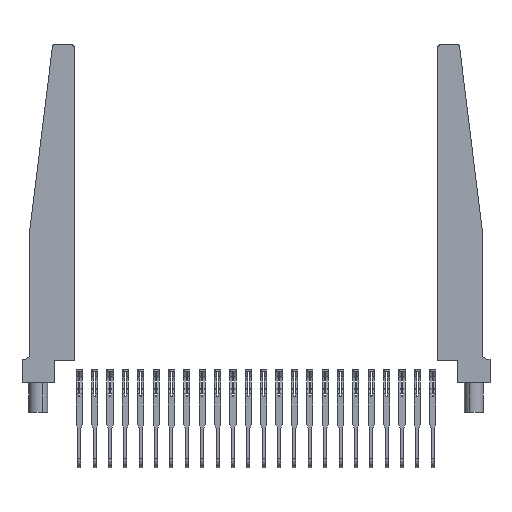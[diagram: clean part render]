
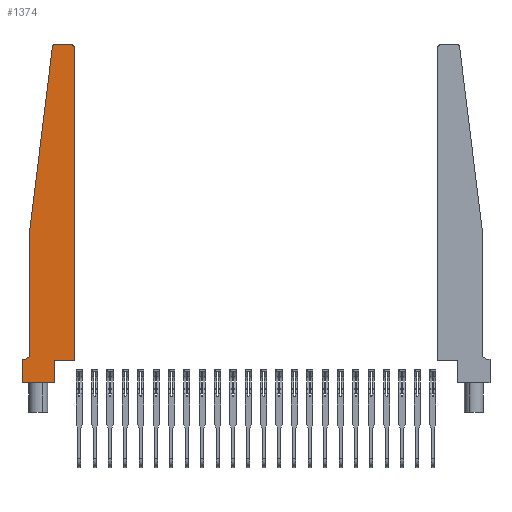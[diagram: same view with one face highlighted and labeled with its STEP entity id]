
A CAD part, top view. The second image highlights one B-rep face of the part: STEP entity #1374.
In plain terms, the highlighted planar face has unit normal (0, 0, 1).
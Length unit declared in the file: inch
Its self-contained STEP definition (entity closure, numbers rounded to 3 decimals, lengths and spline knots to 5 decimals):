
#217 = ORIENTED_EDGE ( 'NONE', *, *, #5809, .T. ) ;
#319 = LINE ( 'NONE', #12160, #12719 ) ;
#435 = CIRCLE ( 'NONE', #21368, 0.03 ) ;
#450 = EDGE_CURVE ( 'NONE', #17572, #12977, #7621, .T. ) ;
#714 = DIRECTION ( 'NONE',  ( -1., 0., 0. ) ) ;
#967 = VERTEX_POINT ( 'NONE', #6766 ) ;
#1080 = DIRECTION ( 'NONE',  ( 1., 0., 0. ) ) ;
#1260 = DIRECTION ( 'NONE',  ( 0., -1., 0. ) ) ;
#1374 = ADVANCED_FACE ( 'NONE', ( #8361 ), #20442, .T. ) ;
#1452 = DIRECTION ( 'NONE',  ( 1., 0., 0. ) ) ;
#1830 = CARTESIAN_POINT ( 'NONE',  ( 0.015, 0.2375, 0.37 ) ) ;
#2026 = ORIENTED_EDGE ( 'NONE', *, *, #15828, .T. ) ;
#2088 = DIRECTION ( 'NONE',  ( -1., 0., 0. ) ) ;
#2246 = CARTESIAN_POINT ( 'NONE',  ( 0.065, 1.25, 0.37 ) ) ;
#2315 = CARTESIAN_POINT ( 'NONE',  ( 0.065, 0.1875, 0.37 ) ) ;
#2542 = VECTOR ( 'NONE', #1260, 39.37008 ) ;
#2791 = LINE ( 'NONE', #9818, #12772 ) ;
#2823 = LINE ( 'NONE', #18687, #9390 ) ;
#3141 = EDGE_CURVE ( 'NONE', #12977, #4894, #17207, .T. ) ;
#3918 = VERTEX_POINT ( 'NONE', #22026 ) ;
#4113 = EDGE_CURVE ( 'NONE', #21723, #4563, #15552, .T. ) ;
#4232 = AXIS2_PLACEMENT_3D ( 'NONE', #1830, #17816, #5049 ) ;
#4384 = ORIENTED_EDGE ( 'NONE', *, *, #6050, .T. ) ;
#4492 = DIRECTION ( 'NONE',  ( 0., 0., 1. ) ) ;
#4563 = VERTEX_POINT ( 'NONE', #21632 ) ;
#4652 = ORIENTED_EDGE ( 'NONE', *, *, #8075, .T. ) ;
#4852 = AXIS2_PLACEMENT_3D ( 'NONE', #13099, #16649, #6331 ) ;
#4894 = VERTEX_POINT ( 'NONE', #12355 ) ;
#5049 = DIRECTION ( 'NONE',  ( -1., 0., 0. ) ) ;
#5094 = DIRECTION ( 'NONE',  ( 1., 0., 0. ) ) ;
#5099 = EDGE_CURVE ( 'NONE', #4563, #3918, #10630, .T. ) ;
#5234 = DIRECTION ( 'NONE',  ( -0.122, -0.992, 0. ) ) ;
#5555 = LINE ( 'NONE', #17849, #11280 ) ;
#5809 = EDGE_CURVE ( 'NONE', #21485, #18608, #18419, .T. ) ;
#6050 = EDGE_CURVE ( 'NONE', #19010, #16733, #435, .T. ) ;
#6229 = ORIENTED_EDGE ( 'NONE', *, *, #4113, .T. ) ;
#6251 = VECTOR ( 'NONE', #12324, 39.37008 ) ;
#6331 = DIRECTION ( 'NONE',  ( 1., 0., 0. ) ) ;
#6519 = DIRECTION ( 'NONE',  ( 0., 0., 1. ) ) ;
#6766 = CARTESIAN_POINT ( 'NONE',  ( 0.065, 1.25, 0.37 ) ) ;
#7621 = LINE ( 'NONE', #2315, #18250 ) ;
#7762 = CARTESIAN_POINT ( 'NONE',  ( 0.425, 2.72, 0.37 ) ) ;
#7809 = ORIENTED_EDGE ( 'NONE', *, *, #5099, .T. ) ;
#7885 = CIRCLE ( 'NONE', #4232, 0.05 ) ;
#8075 = EDGE_CURVE ( 'NONE', #967, #15615, #18000, .T. ) ;
#8361 = FACE_OUTER_BOUND ( 'NONE', #16628, .T. ) ;
#8394 = CARTESIAN_POINT ( 'NONE',  ( 0.395, 2.72, 0.37 ) ) ;
#9390 = VECTOR ( 'NONE', #5234, 39.37008 ) ;
#9399 = CARTESIAN_POINT ( 'NONE',  ( 0.065, 0.2375, 0.37 ) ) ;
#9818 = CARTESIAN_POINT ( 'NONE',  ( 0., 0., 0.37 ) ) ;
#10630 = LINE ( 'NONE', #21315, #22434 ) ;
#10653 = CARTESIAN_POINT ( 'NONE',  ( 0.2605, 0., 0.37 ) ) ;
#10969 = AXIS2_PLACEMENT_3D ( 'NONE', #15249, #6519, #1452 ) ;
#11280 = VECTOR ( 'NONE', #2088, 39.37008 ) ;
#12160 = CARTESIAN_POINT ( 'NONE',  ( 0.425, 0.18, 0.37 ) ) ;
#12324 = DIRECTION ( 'NONE',  ( 0., 1., 0. ) ) ;
#12349 = CARTESIAN_POINT ( 'NONE',  ( 0., 0.1875, 0.37 ) ) ;
#12355 = CARTESIAN_POINT ( 'NONE',  ( 0., 0., 0.37 ) ) ;
#12719 = VECTOR ( 'NONE', #13869, 39.37008 ) ;
#12772 = VECTOR ( 'NONE', #1080, 39.37008 ) ;
#12912 = VECTOR ( 'NONE', #18118, 39.37008 ) ;
#12977 = VERTEX_POINT ( 'NONE', #12349 ) ;
#13099 = CARTESIAN_POINT ( 'NONE',  ( 0.27653, 2.72, 0.37 ) ) ;
#13869 = DIRECTION ( 'NONE',  ( 0., 1., 0. ) ) ;
#14852 = CARTESIAN_POINT ( 'NONE',  ( 0.015, 0.1875, 0.37 ) ) ;
#15009 = ORIENTED_EDGE ( 'NONE', *, *, #17549, .T. ) ;
#15045 = EDGE_CURVE ( 'NONE', #15615, #17572, #7885, .T. ) ;
#15249 = CARTESIAN_POINT ( 'NONE',  ( 0., 0.1875, 0.37 ) ) ;
#15393 = DIRECTION ( 'NONE',  ( 1., 0., 0. ) ) ;
#15552 = LINE ( 'NONE', #17742, #6251 ) ;
#15615 = VERTEX_POINT ( 'NONE', #9399 ) ;
#15654 = ORIENTED_EDGE ( 'NONE', *, *, #17753, .T. ) ;
#15828 = EDGE_CURVE ( 'NONE', #18608, #967, #2823, .T. ) ;
#16628 = EDGE_LOOP ( 'NONE', ( #15009, #217, #2026, #4652, #22563, #20860, #21377, #21407, #6229, #7809, #15654, #4384 ) ) ;
#16649 = DIRECTION ( 'NONE',  ( 0., 0., 1. ) ) ;
#16733 = VERTEX_POINT ( 'NONE', #18125 ) ;
#16983 = CARTESIAN_POINT ( 'NONE',  ( 0., 0., 0.37 ) ) ;
#17207 = LINE ( 'NONE', #16983, #2542 ) ;
#17549 = EDGE_CURVE ( 'NONE', #16733, #21485, #5555, .T. ) ;
#17572 = VERTEX_POINT ( 'NONE', #14852 ) ;
#17742 = CARTESIAN_POINT ( 'NONE',  ( 0.2605, 0.18, 0.37 ) ) ;
#17753 = EDGE_CURVE ( 'NONE', #3918, #19010, #319, .T. ) ;
#17816 = DIRECTION ( 'NONE',  ( 0., 0., -1. ) ) ;
#17849 = CARTESIAN_POINT ( 'NONE',  ( 0.25, 2.75, 0.37 ) ) ;
#18000 = LINE ( 'NONE', #2246, #12912 ) ;
#18118 = DIRECTION ( 'NONE',  ( 0., -1., 0. ) ) ;
#18125 = CARTESIAN_POINT ( 'NONE',  ( 0.395, 2.75, 0.37 ) ) ;
#18250 = VECTOR ( 'NONE', #714, 39.37008 ) ;
#18419 = CIRCLE ( 'NONE', #4852, 0.03 ) ;
#18608 = VERTEX_POINT ( 'NONE', #20659 ) ;
#18687 = CARTESIAN_POINT ( 'NONE',  ( 0.065, 1.25, 0.37 ) ) ;
#18692 = CARTESIAN_POINT ( 'NONE',  ( 0.27653, 2.75, 0.37 ) ) ;
#19010 = VERTEX_POINT ( 'NONE', #7762 ) ;
#19164 = EDGE_CURVE ( 'NONE', #4894, #21723, #2791, .T. ) ;
#20442 = PLANE ( 'NONE',  #10969 ) ;
#20659 = CARTESIAN_POINT ( 'NONE',  ( 0.24675, 2.72367, 0.37 ) ) ;
#20860 = ORIENTED_EDGE ( 'NONE', *, *, #450, .T. ) ;
#21315 = CARTESIAN_POINT ( 'NONE',  ( 0.425, 0.18, 0.37 ) ) ;
#21368 = AXIS2_PLACEMENT_3D ( 'NONE', #8394, #4492, #15393 ) ;
#21377 = ORIENTED_EDGE ( 'NONE', *, *, #3141, .T. ) ;
#21407 = ORIENTED_EDGE ( 'NONE', *, *, #19164, .T. ) ;
#21485 = VERTEX_POINT ( 'NONE', #18692 ) ;
#21632 = CARTESIAN_POINT ( 'NONE',  ( 0.2605, 0.18, 0.37 ) ) ;
#21723 = VERTEX_POINT ( 'NONE', #10653 ) ;
#22026 = CARTESIAN_POINT ( 'NONE',  ( 0.425, 0.18, 0.37 ) ) ;
#22434 = VECTOR ( 'NONE', #5094, 39.37008 ) ;
#22563 = ORIENTED_EDGE ( 'NONE', *, *, #15045, .T. ) ;
